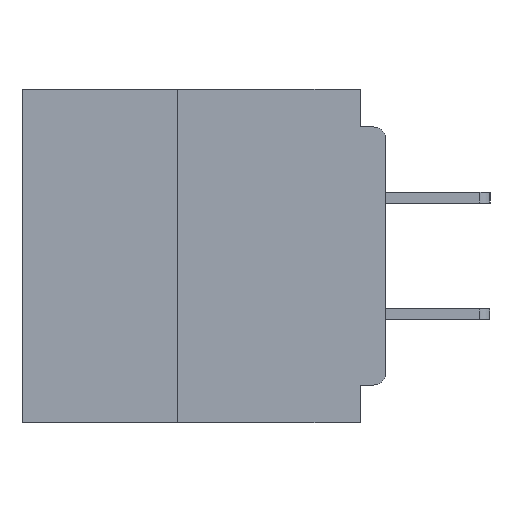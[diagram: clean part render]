
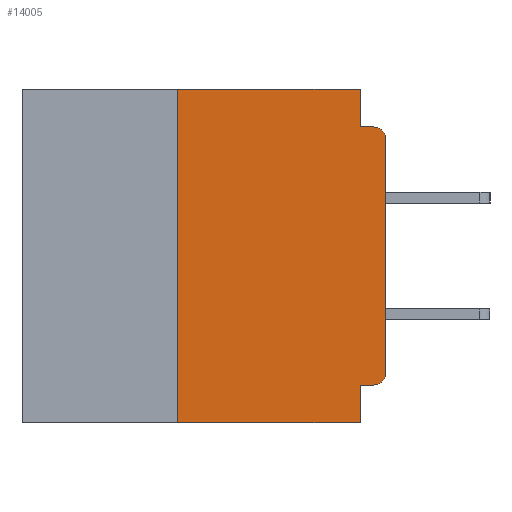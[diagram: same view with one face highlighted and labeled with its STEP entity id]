
A CAD part, left-side view. The second image highlights one B-rep face of the part: STEP entity #14005.
In plain terms, the highlighted planar face has unit normal (-1, 0, 0).
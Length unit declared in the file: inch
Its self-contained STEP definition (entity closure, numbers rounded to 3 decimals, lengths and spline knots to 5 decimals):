
#168 = DIRECTION ( 'NONE',  ( 0., 0., 1. ) ) ;
#830 = LINE ( 'NONE', #51975, #10737 ) ;
#1697 = DIRECTION ( 'NONE',  ( 0., 0., -1. ) ) ;
#1889 = DIRECTION ( 'NONE',  ( 0., -1., 0. ) ) ;
#3022 = AXIS2_PLACEMENT_3D ( 'NONE', #51787, #26902, #1697 ) ;
#3286 = DIRECTION ( 'NONE',  ( 0., -1., 0. ) ) ;
#3510 = VERTEX_POINT ( 'NONE', #22674 ) ;
#3948 = EDGE_CURVE ( 'NONE', #40907, #12787, #17065, .T. ) ;
#3987 = ORIENTED_EDGE ( 'NONE', *, *, #30898, .T. ) ;
#5647 = VERTEX_POINT ( 'NONE', #24291 ) ;
#5705 = LINE ( 'NONE', #33049, #36511 ) ;
#6730 = ORIENTED_EDGE ( 'NONE', *, *, #43307, .T. ) ;
#6826 = CARTESIAN_POINT ( 'NONE',  ( 0., 0.031, -0.045 ) ) ;
#7465 = VERTEX_POINT ( 'NONE', #40660 ) ;
#9313 = CARTESIAN_POINT ( 'NONE',  ( 0., 0.015, -0.045 ) ) ;
#9510 = AXIS2_PLACEMENT_3D ( 'NONE', #35496, #47854, #10462 ) ;
#9907 = CARTESIAN_POINT ( 'NONE',  ( 0., 0.031, 0. ) ) ;
#10047 = EDGE_CURVE ( 'NONE', #27861, #23628, #41042, .T. ) ;
#10462 = DIRECTION ( 'NONE',  ( 0., 0., -1. ) ) ;
#10737 = VECTOR ( 'NONE', #1889, 39.37008 ) ;
#10915 = ORIENTED_EDGE ( 'NONE', *, *, #10047, .F. ) ;
#11118 = CARTESIAN_POINT ( 'NONE',  ( 0., 0.031, -0.4 ) ) ;
#11358 = EDGE_CURVE ( 'NONE', #5647, #7465, #29199, .T. ) ;
#11618 = VERTEX_POINT ( 'NONE', #47886 ) ;
#12361 = CARTESIAN_POINT ( 'NONE',  ( 0., 0., -0.355 ) ) ;
#12787 = VERTEX_POINT ( 'NONE', #30133 ) ;
#13732 = VECTOR ( 'NONE', #25814, 39.37008 ) ;
#14005 = ADVANCED_FACE ( 'NONE', ( #27055 ), #31291, .F. ) ;
#14557 = VECTOR ( 'NONE', #39647, 39.37008 ) ;
#14943 = VECTOR ( 'NONE', #52153, 39.37008 ) ;
#15792 = ORIENTED_EDGE ( 'NONE', *, *, #19158, .F. ) ;
#17065 = LINE ( 'NONE', #12361, #48986 ) ;
#18105 = VECTOR ( 'NONE', #168, 39.37008 ) ;
#18389 = VERTEX_POINT ( 'NONE', #9907 ) ;
#19158 = EDGE_CURVE ( 'NONE', #18389, #27861, #28312, .T. ) ;
#19263 = CARTESIAN_POINT ( 'NONE',  ( 0., 0.015, -0.355 ) ) ;
#19585 = CARTESIAN_POINT ( 'NONE',  ( 0., 0.015, -0.34 ) ) ;
#20094 = VERTEX_POINT ( 'NONE', #11118 ) ;
#20492 = DIRECTION ( 'NONE',  ( 0., 0., -1. ) ) ;
#21599 = CARTESIAN_POINT ( 'NONE',  ( 0., 0.437, 0. ) ) ;
#22674 = CARTESIAN_POINT ( 'NONE',  ( 0., 0.25, 0. ) ) ;
#23075 = CARTESIAN_POINT ( 'NONE',  ( 0., 0.25, -0.4 ) ) ;
#23628 = VERTEX_POINT ( 'NONE', #9313 ) ;
#23834 = DIRECTION ( 'NONE',  ( 0., 0., -1. ) ) ;
#24291 = CARTESIAN_POINT ( 'NONE',  ( 0., 0., -0.34 ) ) ;
#25175 = AXIS2_PLACEMENT_3D ( 'NONE', #19585, #48724, #23834 ) ;
#25814 = DIRECTION ( 'NONE',  ( 0., -1., 0. ) ) ;
#26902 = DIRECTION ( 'NONE',  ( -1., 0., 0. ) ) ;
#27055 = FACE_OUTER_BOUND ( 'NONE', #40070, .T. ) ;
#27861 = VERTEX_POINT ( 'NONE', #6826 ) ;
#28312 = LINE ( 'NONE', #39818, #14557 ) ;
#28956 = CIRCLE ( 'NONE', #3022, 0.015 ) ;
#29062 = EDGE_CURVE ( 'NONE', #11618, #3510, #46878, .T. ) ;
#29199 = LINE ( 'NONE', #29361, #18105 ) ;
#29361 = CARTESIAN_POINT ( 'NONE',  ( 0., 0., 0. ) ) ;
#29860 = ORIENTED_EDGE ( 'NONE', *, *, #48515, .F. ) ;
#30133 = CARTESIAN_POINT ( 'NONE',  ( 0., 0.031, -0.355 ) ) ;
#30898 = EDGE_CURVE ( 'NONE', #7465, #23628, #28956, .T. ) ;
#31291 = PLANE ( 'NONE',  #9510 ) ;
#33049 = CARTESIAN_POINT ( 'NONE',  ( 0., 0.031, -0.4 ) ) ;
#35496 = CARTESIAN_POINT ( 'NONE',  ( 0., 0.437, 0. ) ) ;
#36511 = VECTOR ( 'NONE', #20492, 39.37008 ) ;
#36800 = ORIENTED_EDGE ( 'NONE', *, *, #3948, .F. ) ;
#37862 = ORIENTED_EDGE ( 'NONE', *, *, #41439, .T. ) ;
#38422 = VECTOR ( 'NONE', #3286, 39.37008 ) ;
#38717 = EDGE_CURVE ( 'NONE', #3510, #18389, #46970, .T. ) ;
#39647 = DIRECTION ( 'NONE',  ( 0., 0., -1. ) ) ;
#39818 = CARTESIAN_POINT ( 'NONE',  ( 0., 0.031, 0. ) ) ;
#40070 = EDGE_LOOP ( 'NONE', ( #45978, #3987, #10915, #15792, #48021, #45093, #37862, #29860, #36800, #6730 ) ) ;
#40660 = CARTESIAN_POINT ( 'NONE',  ( 0., 0., -0.06 ) ) ;
#40907 = VERTEX_POINT ( 'NONE', #19263 ) ;
#41042 = LINE ( 'NONE', #44999, #38422 ) ;
#41439 = EDGE_CURVE ( 'NONE', #11618, #20094, #830, .T. ) ;
#41895 = DIRECTION ( 'NONE',  ( 0., 1., 0. ) ) ;
#43307 = EDGE_CURVE ( 'NONE', #40907, #5647, #50416, .T. ) ;
#44999 = CARTESIAN_POINT ( 'NONE',  ( 0., 0., -0.045 ) ) ;
#45093 = ORIENTED_EDGE ( 'NONE', *, *, #29062, .F. ) ;
#45978 = ORIENTED_EDGE ( 'NONE', *, *, #11358, .T. ) ;
#46878 = LINE ( 'NONE', #23075, #14943 ) ;
#46970 = LINE ( 'NONE', #21599, #13732 ) ;
#47854 = DIRECTION ( 'NONE',  ( 1., 0., 0. ) ) ;
#47886 = CARTESIAN_POINT ( 'NONE',  ( 0., 0.25, -0.4 ) ) ;
#48021 = ORIENTED_EDGE ( 'NONE', *, *, #38717, .F. ) ;
#48515 = EDGE_CURVE ( 'NONE', #12787, #20094, #5705, .T. ) ;
#48724 = DIRECTION ( 'NONE',  ( -1., 0., 0. ) ) ;
#48986 = VECTOR ( 'NONE', #41895, 39.37008 ) ;
#50416 = CIRCLE ( 'NONE', #25175, 0.015 ) ;
#51787 = CARTESIAN_POINT ( 'NONE',  ( 0., 0.015, -0.06 ) ) ;
#51975 = CARTESIAN_POINT ( 'NONE',  ( 0., 0.437, -0.4 ) ) ;
#52153 = DIRECTION ( 'NONE',  ( 0., 0., 1. ) ) ;
